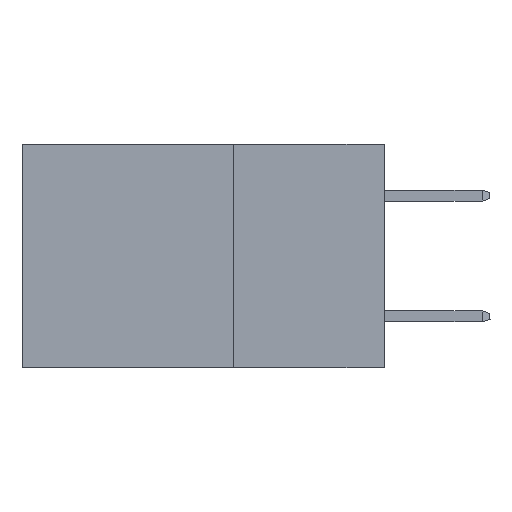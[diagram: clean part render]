
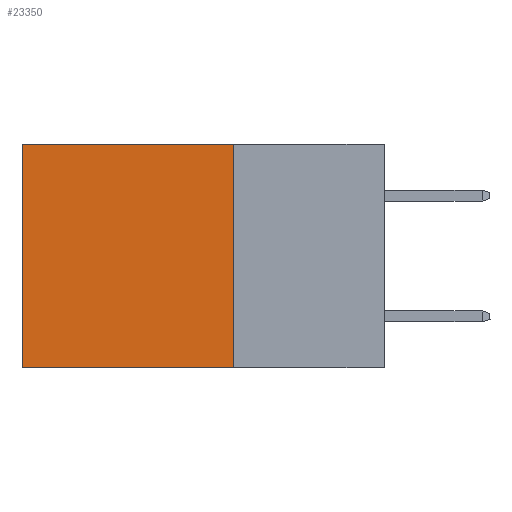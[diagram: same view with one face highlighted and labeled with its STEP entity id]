
A CAD part, left-side view. The second image highlights one B-rep face of the part: STEP entity #23350.
In plain terms, the highlighted planar face has unit normal (-1, 0, 0).
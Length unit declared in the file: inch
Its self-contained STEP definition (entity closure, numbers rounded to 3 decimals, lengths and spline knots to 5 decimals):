
#937 = DIRECTION ( 'NONE',  ( 0., 0., -1. ) ) ;
#1917 = CARTESIAN_POINT ( 'NONE',  ( 0.2615, 0.6, -0.37 ) ) ;
#3253 = VECTOR ( 'NONE', #7881, 39.37008 ) ;
#3517 = EDGE_CURVE ( 'NONE', #10623, #9946, #7400, .T. ) ;
#3807 = EDGE_CURVE ( 'NONE', #9386, #9946, #5251, .T. ) ;
#4129 = PLANE ( 'NONE',  #13270 ) ;
#4890 = CARTESIAN_POINT ( 'NONE',  ( 0.2615, 0.25, -0.37 ) ) ;
#5251 = LINE ( 'NONE', #22063, #15015 ) ;
#6076 = DIRECTION ( 'NONE',  ( 1., 0., 0. ) ) ;
#6956 = CARTESIAN_POINT ( 'NONE',  ( 0.2615, 0.25, 0. ) ) ;
#7400 = LINE ( 'NONE', #1917, #17103 ) ;
#7799 = CARTESIAN_POINT ( 'NONE',  ( 0.2615, 0.25, -0.37 ) ) ;
#7881 = DIRECTION ( 'NONE',  ( 0., 0., -1. ) ) ;
#7996 = LINE ( 'NONE', #12970, #22804 ) ;
#8826 = ORIENTED_EDGE ( 'NONE', *, *, #21456, .T. ) ;
#9386 = VERTEX_POINT ( 'NONE', #4890 ) ;
#9946 = VERTEX_POINT ( 'NONE', #10871 ) ;
#10062 = CARTESIAN_POINT ( 'NONE',  ( 0.2615, 0.6, 0. ) ) ;
#10623 = VERTEX_POINT ( 'NONE', #10062 ) ;
#10871 = CARTESIAN_POINT ( 'NONE',  ( 0.2615, 0.6, -0.37 ) ) ;
#10918 = VERTEX_POINT ( 'NONE', #6956 ) ;
#11895 = CARTESIAN_POINT ( 'NONE',  ( 0.2615, 0.25, -0.37 ) ) ;
#12970 = CARTESIAN_POINT ( 'NONE',  ( 0.2615, 0.25, 0. ) ) ;
#13270 = AXIS2_PLACEMENT_3D ( 'NONE', #11895, #6076, #19637 ) ;
#13868 = ORIENTED_EDGE ( 'NONE', *, *, #3807, .F. ) ;
#14052 = ORIENTED_EDGE ( 'NONE', *, *, #3517, .T. ) ;
#15015 = VECTOR ( 'NONE', #21995, 39.37008 ) ;
#16290 = FACE_OUTER_BOUND ( 'NONE', #17608, .T. ) ;
#17103 = VECTOR ( 'NONE', #937, 39.37008 ) ;
#17608 = EDGE_LOOP ( 'NONE', ( #14052, #13868, #18546, #8826 ) ) ;
#18546 = ORIENTED_EDGE ( 'NONE', *, *, #22421, .F. ) ;
#18717 = LINE ( 'NONE', #7799, #3253 ) ;
#19637 = DIRECTION ( 'NONE',  ( 0., 0., -1. ) ) ;
#20708 = DIRECTION ( 'NONE',  ( 0., 1., 0. ) ) ;
#21456 = EDGE_CURVE ( 'NONE', #10918, #10623, #7996, .T. ) ;
#21995 = DIRECTION ( 'NONE',  ( 0., 1., 0. ) ) ;
#22063 = CARTESIAN_POINT ( 'NONE',  ( 0.2615, 0.25, -0.37 ) ) ;
#22421 = EDGE_CURVE ( 'NONE', #10918, #9386, #18717, .T. ) ;
#22804 = VECTOR ( 'NONE', #20708, 39.37008 ) ;
#23350 = ADVANCED_FACE ( 'NONE', ( #16290 ), #4129, .F. ) ;
